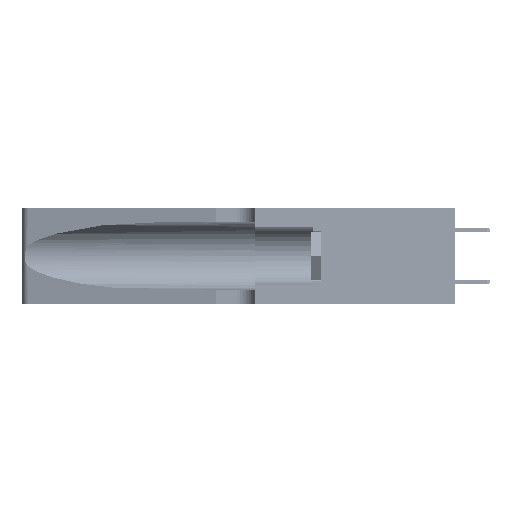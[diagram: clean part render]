
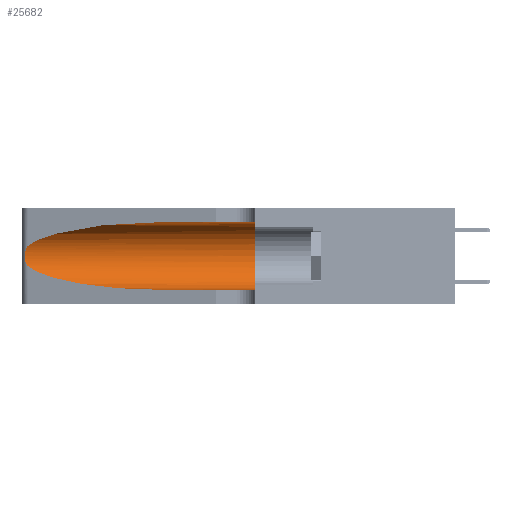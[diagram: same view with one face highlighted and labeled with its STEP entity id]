
A CAD part, left-side view. The second image highlights one B-rep face of the part: STEP entity #25682.
In plain terms, the highlighted cylindrical face has radius 3.308 mm (diameter 6.617 mm), a partial arc.
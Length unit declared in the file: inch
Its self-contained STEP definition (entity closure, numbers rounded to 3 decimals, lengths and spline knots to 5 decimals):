
#2588 = CARTESIAN_POINT ( 'NONE',  ( 0.18966, 0.96281, 0.31525 ) ) ;
#3023 =( BOUNDED_CURVE ( )  B_SPLINE_CURVE ( 3, ( #36207, #36468, #16281, #27677 ),
 .UNSPECIFIED., .F., .T. ) 
 B_SPLINE_CURVE_WITH_KNOTS ( ( 4, 4 ),
 ( 3.44316, 4.71239 ),
 .UNSPECIFIED. ) 
 CURVE ( )  GEOMETRIC_REPRESENTATION_ITEM ( )  RATIONAL_B_SPLINE_CURVE ( ( 1., 0.87, 0.87, 1. ) ) 
 REPRESENTATION_ITEM ( '' )  );
#3339 =( BOUNDED_CURVE ( )  B_SPLINE_CURVE ( 3, ( #41800, #2588, #6209, #37715 ),
 .UNSPECIFIED., .F., .T. ) 
 B_SPLINE_CURVE_WITH_KNOTS ( ( 4, 4 ),
 ( 1.5708, 2.84003 ),
 .UNSPECIFIED. ) 
 CURVE ( )  GEOMETRIC_REPRESENTATION_ITEM ( )  RATIONAL_B_SPLINE_CURVE ( ( 1., 0.87, 0.87, 1. ) ) 
 REPRESENTATION_ITEM ( '' )  );
#3362 = CARTESIAN_POINT ( 'NONE',  ( 0.25487, 1.22718, 0.22369 ) ) ;
#4388 = CARTESIAN_POINT ( 'NONE',  ( 0.25639, 1.23186, 0.15144 ) ) ;
#5923 = AXIS2_PLACEMENT_3D ( 'NONE', #23546, #8833, #36491 ) ;
#6209 = CARTESIAN_POINT ( 'NONE',  ( 0.2373, 1.15595, 0.28018 ) ) ;
#6438 = CARTESIAN_POINT ( 'NONE',  ( 0.1305, 0.35, 0.05475 ) ) ;
#7486 = CARTESIAN_POINT ( 'NONE',  ( 0.25555, 1.22994, 0.2215 ) ) ;
#7737 = CARTESIAN_POINT ( 'NONE',  ( 0.25787, 1.23484, 0.2124 ) ) ;
#8729 = DIRECTION ( 'NONE',  ( 0., -1., 0. ) ) ;
#8747 = CARTESIAN_POINT ( 'NONE',  ( 0.26017, 1.23833, 0.17102 ) ) ;
#8833 = DIRECTION ( 'NONE',  ( 0., 1., 0. ) ) ;
#10924 = EDGE_CURVE ( 'NONE', #40211, #28993, #3023, .T. ) ;
#14390 = ORIENTED_EDGE ( 'NONE', *, *, #10924, .T. ) ;
#15780 = CARTESIAN_POINT ( 'NONE',  ( 0.25487, 1.22718, 0.14631 ) ) ;
#16281 = CARTESIAN_POINT ( 'NONE',  ( 0.18966, 0.96281, 0.05475 ) ) ;
#16714 = CARTESIAN_POINT ( 'NONE',  ( 0.25487, 1.22718, 0.14631 ) ) ;
#17216 = CARTESIAN_POINT ( 'NONE',  ( 0.25856, 1.23593, 0.16098 ) ) ;
#21546 = CIRCLE ( 'NONE', #5923, 0.13025 ) ;
#22430 = LINE ( 'NONE', #45434, #47795 ) ;
#22635 = VERTEX_POINT ( 'NONE', #6438 ) ;
#23198 = CARTESIAN_POINT ( 'NONE',  ( 0.25639, 1.23184, 0.21858 ) ) ;
#23546 = CARTESIAN_POINT ( 'NONE',  ( 0.1305, 0.35, 0.185 ) ) ;
#23965 = CARTESIAN_POINT ( 'NONE',  ( 0.26075, 1.23896, 0.178 ) ) ;
#24226 = CARTESIAN_POINT ( 'NONE',  ( 0.25555, 1.22993, 0.14849 ) ) ;
#25203 = CARTESIAN_POINT ( 'NONE',  ( 0.1305, 1.61858, 0.31525 ) ) ;
#25485 = EDGE_CURVE ( 'NONE', #29034, #40211, #27100, .T. ) ;
#25599 = AXIS2_PLACEMENT_3D ( 'NONE', #29367, #44845, #34028 ) ;
#25682 = ADVANCED_FACE ( 'NONE', ( #33258 ), #41982, .F. ) ;
#26481 = ORIENTED_EDGE ( 'NONE', *, *, #26639, .T. ) ;
#26639 = EDGE_CURVE ( 'NONE', #28993, #22635, #22430, .T. ) ;
#27100 = B_SPLINE_CURVE_WITH_KNOTS ( 'NONE', 3,
 ( #3362, #7486, #23198, #7737, #28849, #48186, #44580, #23965, #8747, #17216, #40232, #4388, #24226, #16714 ),
 .UNSPECIFIED., .F., .F.,
 ( 4, 2, 2, 2, 2, 2, 4 ),
 ( 0., 0.00027, 0.00053, 0.00107, 0.0016, 0.00187, 0.00214 ),
 .UNSPECIFIED. ) ;
#27208 = VECTOR ( 'NONE', #8729, 39.37008 ) ;
#27677 = CARTESIAN_POINT ( 'NONE',  ( 0.1305, 0.72297, 0.05475 ) ) ;
#28849 = CARTESIAN_POINT ( 'NONE',  ( 0.25854, 1.2359, 0.20912 ) ) ;
#28993 = VERTEX_POINT ( 'NONE', #42439 ) ;
#29034 = VERTEX_POINT ( 'NONE', #42689 ) ;
#29367 = CARTESIAN_POINT ( 'NONE',  ( 0.1305, 1.61858, 0.185 ) ) ;
#30146 = EDGE_LOOP ( 'NONE', ( #35414, #44250, #14390, #26481, #36080, #50048 ) ) ;
#31373 = VERTEX_POINT ( 'NONE', #46686 ) ;
#33258 = FACE_OUTER_BOUND ( 'NONE', #30146, .T. ) ;
#34028 = DIRECTION ( 'NONE',  ( 0., 0., -1. ) ) ;
#35155 = EDGE_CURVE ( 'NONE', #31373, #29034, #3339, .T. ) ;
#35414 = ORIENTED_EDGE ( 'NONE', *, *, #35155, .T. ) ;
#36080 = ORIENTED_EDGE ( 'NONE', *, *, #46175, .F. ) ;
#36207 = CARTESIAN_POINT ( 'NONE',  ( 0.25487, 1.22718, 0.14631 ) ) ;
#36468 = CARTESIAN_POINT ( 'NONE',  ( 0.2373, 1.15595, 0.08982 ) ) ;
#36491 = DIRECTION ( 'NONE',  ( 0., 0., 1. ) ) ;
#37715 = CARTESIAN_POINT ( 'NONE',  ( 0.25487, 1.22718, 0.22369 ) ) ;
#40211 = VERTEX_POINT ( 'NONE', #15780 ) ;
#40232 = CARTESIAN_POINT ( 'NONE',  ( 0.25789, 1.23486, 0.15765 ) ) ;
#41800 = CARTESIAN_POINT ( 'NONE',  ( 0.1305, 0.72297, 0.31525 ) ) ;
#41982 = CYLINDRICAL_SURFACE ( 'NONE', #25599, 0.13025 ) ;
#42439 = CARTESIAN_POINT ( 'NONE',  ( 0.1305, 0.72297, 0.05475 ) ) ;
#42689 = CARTESIAN_POINT ( 'NONE',  ( 0.25487, 1.22718, 0.22369 ) ) ;
#42785 = EDGE_CURVE ( 'NONE', #31373, #50636, #47672, .T. ) ;
#43474 = CARTESIAN_POINT ( 'NONE',  ( 0.1305, 0.35, 0.31525 ) ) ;
#44250 = ORIENTED_EDGE ( 'NONE', *, *, #25485, .T. ) ;
#44580 = CARTESIAN_POINT ( 'NONE',  ( 0.26075, 1.23896, 0.19203 ) ) ;
#44845 = DIRECTION ( 'NONE',  ( 0., -1., 0. ) ) ;
#45434 = CARTESIAN_POINT ( 'NONE',  ( 0.1305, 1.61858, 0.05475 ) ) ;
#46175 = EDGE_CURVE ( 'NONE', #50636, #22635, #21546, .T. ) ;
#46686 = CARTESIAN_POINT ( 'NONE',  ( 0.1305, 0.72297, 0.31525 ) ) ;
#47672 = LINE ( 'NONE', #25203, #27208 ) ;
#47795 = VECTOR ( 'NONE', #49540, 39.37008 ) ;
#48186 = CARTESIAN_POINT ( 'NONE',  ( 0.26018, 1.23835, 0.19895 ) ) ;
#49540 = DIRECTION ( 'NONE',  ( 0., -1., 0. ) ) ;
#50048 = ORIENTED_EDGE ( 'NONE', *, *, #42785, .F. ) ;
#50636 = VERTEX_POINT ( 'NONE', #43474 ) ;
